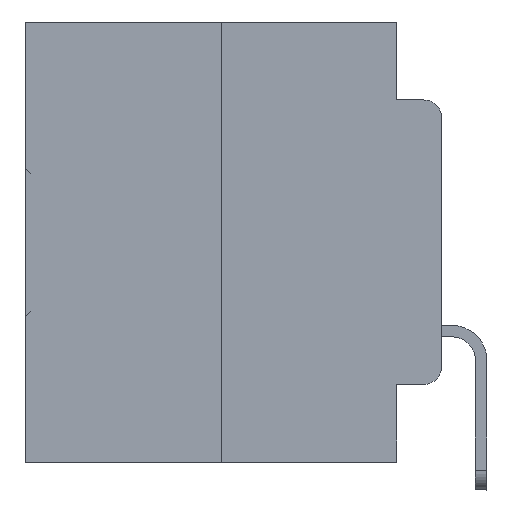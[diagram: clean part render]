
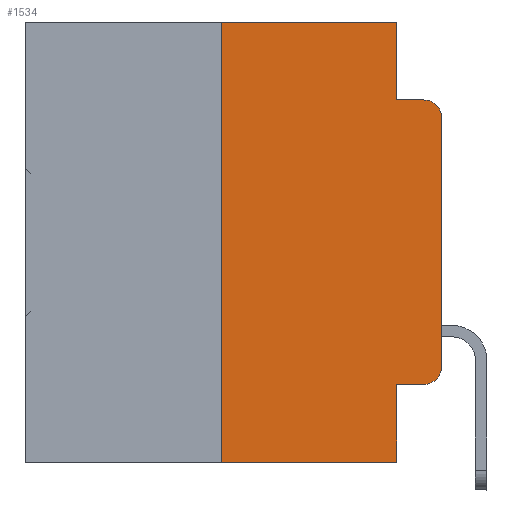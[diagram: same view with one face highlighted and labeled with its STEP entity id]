
A CAD part, left-side view. The second image highlights one B-rep face of the part: STEP entity #1534.
In plain terms, the highlighted planar face has unit normal (-1, 0, 0).
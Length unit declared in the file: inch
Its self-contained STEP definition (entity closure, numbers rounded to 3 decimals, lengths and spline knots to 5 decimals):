
#152 = PLANE ( 'NONE',  #17477 ) ;
#177 = CARTESIAN_POINT ( 'NONE',  ( 0., 0., -0.1085 ) ) ;
#256 = CARTESIAN_POINT ( 'NONE',  ( 0., 0.473, 0. ) ) ;
#1484 = CARTESIAN_POINT ( 'NONE',  ( 0., 0.02, -0.1085 ) ) ;
#1534 = ADVANCED_FACE ( 'NONE', ( #28411 ), #152, .F. ) ;
#1769 = CARTESIAN_POINT ( 'NONE',  ( 0., 0.051, -0.4115 ) ) ;
#1893 = ORIENTED_EDGE ( 'NONE', *, *, #26313, .F. ) ;
#2395 = ORIENTED_EDGE ( 'NONE', *, *, #27035, .F. ) ;
#2858 = DIRECTION ( 'NONE',  ( 0., 0., -1. ) ) ;
#2936 = ORIENTED_EDGE ( 'NONE', *, *, #18191, .T. ) ;
#3140 = EDGE_CURVE ( 'NONE', #8996, #14222, #27164, .T. ) ;
#4140 = CARTESIAN_POINT ( 'NONE',  ( 0., 0.02, -0.0885 ) ) ;
#4326 = CARTESIAN_POINT ( 'NONE',  ( 0., 0.473, 0. ) ) ;
#4636 = CARTESIAN_POINT ( 'NONE',  ( 0., 0.25, 0. ) ) ;
#4642 = AXIS2_PLACEMENT_3D ( 'NONE', #1484, #23508, #16194 ) ;
#5535 = LINE ( 'NONE', #4326, #7862 ) ;
#5746 = VECTOR ( 'NONE', #22584, 39.37008 ) ;
#6763 = DIRECTION ( 'NONE',  ( 0., -1., 0. ) ) ;
#6839 = VECTOR ( 'NONE', #15737, 39.37008 ) ;
#7257 = CARTESIAN_POINT ( 'NONE',  ( 0., 0.051, 0. ) ) ;
#7644 = CARTESIAN_POINT ( 'NONE',  ( 0., 0.051, 0. ) ) ;
#7660 = CARTESIAN_POINT ( 'NONE',  ( 0., 0.051, -0.5 ) ) ;
#7862 = VECTOR ( 'NONE', #14776, 39.37008 ) ;
#8001 = DIRECTION ( 'NONE',  ( 0., 0., -1. ) ) ;
#8996 = VERTEX_POINT ( 'NONE', #22649 ) ;
#9458 = DIRECTION ( 'NONE',  ( 0., 0., 1. ) ) ;
#9688 = VERTEX_POINT ( 'NONE', #7660 ) ;
#10524 = VECTOR ( 'NONE', #31821, 39.37008 ) ;
#11081 = ORIENTED_EDGE ( 'NONE', *, *, #21502, .F. ) ;
#11697 = LINE ( 'NONE', #4636, #10524 ) ;
#11916 = CARTESIAN_POINT ( 'NONE',  ( 0., 0., -0.3915 ) ) ;
#13125 = AXIS2_PLACEMENT_3D ( 'NONE', #14791, #31494, #17395 ) ;
#14222 = VERTEX_POINT ( 'NONE', #4140 ) ;
#14776 = DIRECTION ( 'NONE',  ( 0., -1., 0. ) ) ;
#14791 = CARTESIAN_POINT ( 'NONE',  ( 0., 0.02, -0.3915 ) ) ;
#14905 = EDGE_CURVE ( 'NONE', #28213, #30028, #31384, .T. ) ;
#15185 = ORIENTED_EDGE ( 'NONE', *, *, #26474, .F. ) ;
#15600 = ORIENTED_EDGE ( 'NONE', *, *, #26373, .T. ) ;
#15603 = ORIENTED_EDGE ( 'NONE', *, *, #3140, .F. ) ;
#15737 = DIRECTION ( 'NONE',  ( 0., -1., 0. ) ) ;
#16118 = CIRCLE ( 'NONE', #4642, 0.02 ) ;
#16194 = DIRECTION ( 'NONE',  ( 0., 0., -1. ) ) ;
#16213 = VECTOR ( 'NONE', #22658, 39.37008 ) ;
#17395 = DIRECTION ( 'NONE',  ( 0., 0., -1. ) ) ;
#17477 = AXIS2_PLACEMENT_3D ( 'NONE', #256, #25311, #8001 ) ;
#17563 = LINE ( 'NONE', #7257, #32068 ) ;
#18191 = EDGE_CURVE ( 'NONE', #32300, #28213, #31136, .T. ) ;
#19082 = LINE ( 'NONE', #7644, #5746 ) ;
#19085 = EDGE_CURVE ( 'NONE', #22962, #9688, #31112, .T. ) ;
#19468 = ORIENTED_EDGE ( 'NONE', *, *, #14905, .T. ) ;
#19568 = CARTESIAN_POINT ( 'NONE',  ( 0., 0.051, -0.0885 ) ) ;
#20078 = CARTESIAN_POINT ( 'NONE',  ( 0., 0.25, -0.5 ) ) ;
#20709 = VECTOR ( 'NONE', #9458, 39.37008 ) ;
#21342 = EDGE_LOOP ( 'NONE', ( #15600, #28557, #15603, #15185, #11081, #1893, #22903, #2395, #2936, #19468 ) ) ;
#21502 = EDGE_CURVE ( 'NONE', #24440, #25674, #5535, .T. ) ;
#21991 = EDGE_CURVE ( 'NONE', #24190, #14222, #16118, .T. ) ;
#22111 = CARTESIAN_POINT ( 'NONE',  ( 0., 0.02, -0.4115 ) ) ;
#22584 = DIRECTION ( 'NONE',  ( 0., 0., -1. ) ) ;
#22649 = CARTESIAN_POINT ( 'NONE',  ( 0., 0.051, -0.0885 ) ) ;
#22658 = DIRECTION ( 'NONE',  ( 0., -1., 0. ) ) ;
#22903 = ORIENTED_EDGE ( 'NONE', *, *, #19085, .T. ) ;
#22962 = VERTEX_POINT ( 'NONE', #20078 ) ;
#23508 = DIRECTION ( 'NONE',  ( -1., 0., 0. ) ) ;
#23898 = CARTESIAN_POINT ( 'NONE',  ( 0., 0.25, 0. ) ) ;
#24187 = LINE ( 'NONE', #24463, #20709 ) ;
#24190 = VERTEX_POINT ( 'NONE', #177 ) ;
#24440 = VERTEX_POINT ( 'NONE', #23898 ) ;
#24463 = CARTESIAN_POINT ( 'NONE',  ( 0., 0., 0. ) ) ;
#24616 = CARTESIAN_POINT ( 'NONE',  ( 0., 0.473, -0.5 ) ) ;
#25311 = DIRECTION ( 'NONE',  ( 1., 0., 0. ) ) ;
#25674 = VERTEX_POINT ( 'NONE', #29189 ) ;
#26313 = EDGE_CURVE ( 'NONE', #22962, #24440, #11697, .T. ) ;
#26373 = EDGE_CURVE ( 'NONE', #30028, #24190, #24187, .T. ) ;
#26474 = EDGE_CURVE ( 'NONE', #25674, #8996, #17563, .T. ) ;
#27035 = EDGE_CURVE ( 'NONE', #32300, #9688, #19082, .T. ) ;
#27164 = LINE ( 'NONE', #19568, #16213 ) ;
#28213 = VERTEX_POINT ( 'NONE', #22111 ) ;
#28336 = VECTOR ( 'NONE', #6763, 39.37008 ) ;
#28411 = FACE_OUTER_BOUND ( 'NONE', #21342, .T. ) ;
#28487 = CARTESIAN_POINT ( 'NONE',  ( 0., 0.051, -0.4115 ) ) ;
#28557 = ORIENTED_EDGE ( 'NONE', *, *, #21991, .T. ) ;
#29189 = CARTESIAN_POINT ( 'NONE',  ( 0., 0.051, 0. ) ) ;
#30028 = VERTEX_POINT ( 'NONE', #11916 ) ;
#31112 = LINE ( 'NONE', #24616, #28336 ) ;
#31136 = LINE ( 'NONE', #28487, #6839 ) ;
#31384 = CIRCLE ( 'NONE', #13125, 0.02 ) ;
#31494 = DIRECTION ( 'NONE',  ( -1., 0., 0. ) ) ;
#31821 = DIRECTION ( 'NONE',  ( 0., 0., 1. ) ) ;
#32068 = VECTOR ( 'NONE', #2858, 39.37008 ) ;
#32300 = VERTEX_POINT ( 'NONE', #1769 ) ;
